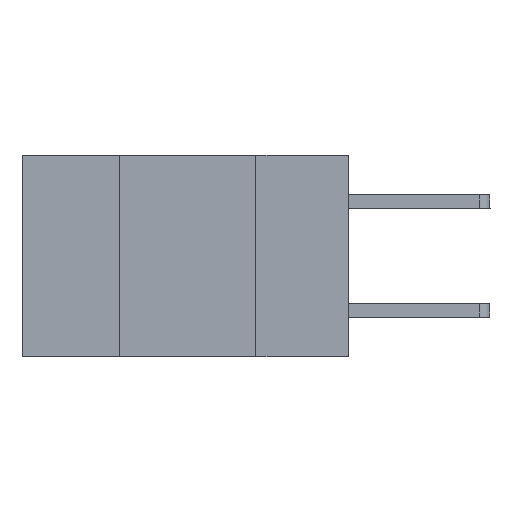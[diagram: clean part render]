
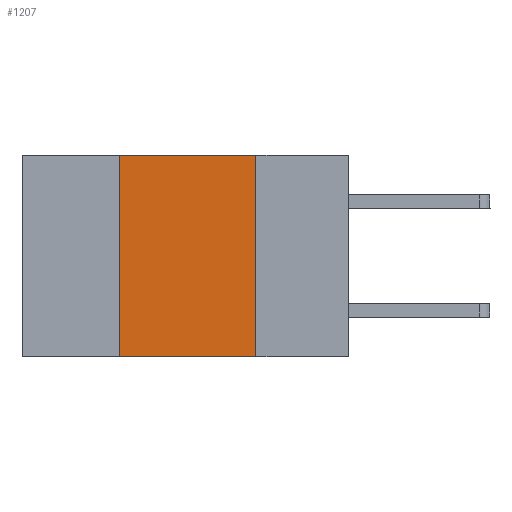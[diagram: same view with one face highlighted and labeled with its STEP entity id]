
A CAD part, left-side view. The second image highlights one B-rep face of the part: STEP entity #1207.
In plain terms, the highlighted planar face has unit normal (-1, 0, 0).
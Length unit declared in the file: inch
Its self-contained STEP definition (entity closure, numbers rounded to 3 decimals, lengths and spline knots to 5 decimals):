
#255 = CARTESIAN_POINT ( 'NONE',  ( 0., 0.42, 0. ) ) ;
#523 = EDGE_CURVE ( 'NONE', #7417, #5139, #2101, .T. ) ;
#631 = DIRECTION ( 'NONE',  ( 0., 0., 1. ) ) ;
#776 = EDGE_CURVE ( 'NONE', #1984, #5139, #8445, .T. ) ;
#1197 = ORIENTED_EDGE ( 'NONE', *, *, #6866, .F. ) ;
#1207 = ADVANCED_FACE ( 'NONE', ( #2352 ), #3016, .F. ) ;
#1304 = CARTESIAN_POINT ( 'NONE',  ( 0., 0.6, -0.37 ) ) ;
#1312 = EDGE_LOOP ( 'NONE', ( #7983, #1197, #7155, #9281 ) ) ;
#1443 = VERTEX_POINT ( 'NONE', #255 ) ;
#1984 = VERTEX_POINT ( 'NONE', #2973 ) ;
#2101 = LINE ( 'NONE', #8001, #8987 ) ;
#2352 = FACE_OUTER_BOUND ( 'NONE', #1312, .T. ) ;
#2807 = LINE ( 'NONE', #8475, #6909 ) ;
#2973 = CARTESIAN_POINT ( 'NONE',  ( 0., 0.42, -0.37 ) ) ;
#3016 = PLANE ( 'NONE',  #4580 ) ;
#3592 = DIRECTION ( 'NONE',  ( 0., -1., 0. ) ) ;
#3623 = DIRECTION ( 'NONE',  ( 0., 0., -1. ) ) ;
#4580 = AXIS2_PLACEMENT_3D ( 'NONE', #8245, #4622, #7540 ) ;
#4622 = DIRECTION ( 'NONE',  ( 1., 0., 0. ) ) ;
#5139 = VERTEX_POINT ( 'NONE', #6212 ) ;
#5733 = DIRECTION ( 'NONE',  ( 0., -1., 0. ) ) ;
#6153 = VECTOR ( 'NONE', #3592, 39.37008 ) ;
#6212 = CARTESIAN_POINT ( 'NONE',  ( 0., 0.17, -0.37 ) ) ;
#6866 = EDGE_CURVE ( 'NONE', #1443, #7417, #9257, .T. ) ;
#6909 = VECTOR ( 'NONE', #631, 39.37008 ) ;
#7109 = CARTESIAN_POINT ( 'NONE',  ( 0., 0.17, 0. ) ) ;
#7155 = ORIENTED_EDGE ( 'NONE', *, *, #7342, .F. ) ;
#7159 = CARTESIAN_POINT ( 'NONE',  ( 0., 0.6, 0. ) ) ;
#7173 = VECTOR ( 'NONE', #5733, 39.37008 ) ;
#7342 = EDGE_CURVE ( 'NONE', #1984, #1443, #2807, .T. ) ;
#7417 = VERTEX_POINT ( 'NONE', #7109 ) ;
#7540 = DIRECTION ( 'NONE',  ( 0., 0., -1. ) ) ;
#7983 = ORIENTED_EDGE ( 'NONE', *, *, #523, .F. ) ;
#8001 = CARTESIAN_POINT ( 'NONE',  ( 0., 0.17, 0. ) ) ;
#8245 = CARTESIAN_POINT ( 'NONE',  ( 0., 0.6, 0. ) ) ;
#8445 = LINE ( 'NONE', #1304, #7173 ) ;
#8475 = CARTESIAN_POINT ( 'NONE',  ( 0., 0.42, 0. ) ) ;
#8987 = VECTOR ( 'NONE', #3623, 39.37008 ) ;
#9257 = LINE ( 'NONE', #7159, #6153 ) ;
#9281 = ORIENTED_EDGE ( 'NONE', *, *, #776, .T. ) ;
